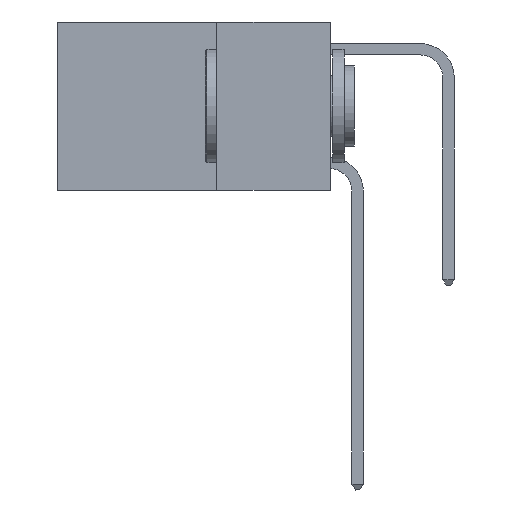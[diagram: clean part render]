
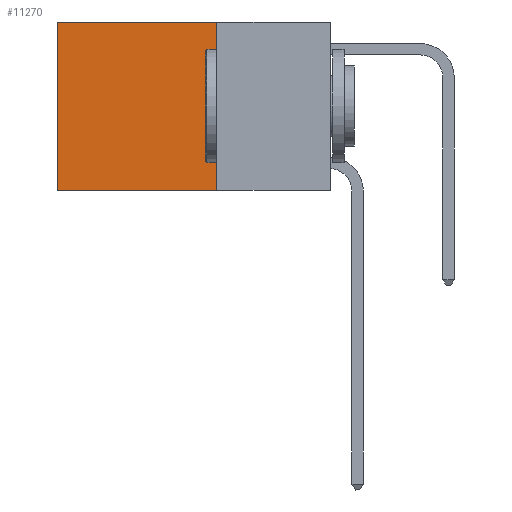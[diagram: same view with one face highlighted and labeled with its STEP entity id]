
A CAD part, left-side view. The second image highlights one B-rep face of the part: STEP entity #11270.
In plain terms, the highlighted planar face has unit normal (-1, 0, 0).
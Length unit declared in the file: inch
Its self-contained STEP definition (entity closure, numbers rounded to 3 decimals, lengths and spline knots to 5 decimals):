
#878 = DIRECTION ( 'NONE',  ( 1., 0., 0. ) ) ;
#1355 = ORIENTED_EDGE ( 'NONE', *, *, #2748, .T. ) ;
#2748 = EDGE_CURVE ( 'NONE', #13776, #4436, #9092, .T. ) ;
#3524 = EDGE_CURVE ( 'NONE', #13776, #14113, #11293, .T. ) ;
#4199 = CARTESIAN_POINT ( 'NONE',  ( 0.2625, 0.25, 0. ) ) ;
#4202 = DIRECTION ( 'NONE',  ( 0., 0., -1. ) ) ;
#4373 = VECTOR ( 'NONE', #18353, 39.37008 ) ;
#4436 = VERTEX_POINT ( 'NONE', #5403 ) ;
#4702 = CARTESIAN_POINT ( 'NONE',  ( 0.2625, 0.6, -0.37 ) ) ;
#5315 = VECTOR ( 'NONE', #4202, 39.37008 ) ;
#5403 = CARTESIAN_POINT ( 'NONE',  ( 0.2625, 0.6, 0. ) ) ;
#5965 = ORIENTED_EDGE ( 'NONE', *, *, #11442, .F. ) ;
#6932 = DIRECTION ( 'NONE',  ( 0., 0., -1. ) ) ;
#7676 = DIRECTION ( 'NONE',  ( 0., 0., -1. ) ) ;
#7707 = ORIENTED_EDGE ( 'NONE', *, *, #3524, .F. ) ;
#8050 = VECTOR ( 'NONE', #8995, 39.37008 ) ;
#8188 = CARTESIAN_POINT ( 'NONE',  ( 0.2625, 0.6, 0. ) ) ;
#8995 = DIRECTION ( 'NONE',  ( 0., 1., 0. ) ) ;
#9092 = LINE ( 'NONE', #9286, #8050 ) ;
#9260 = PLANE ( 'NONE',  #15032 ) ;
#9286 = CARTESIAN_POINT ( 'NONE',  ( 0.2625, 0.25, 0. ) ) ;
#9537 = LINE ( 'NONE', #11020, #4373 ) ;
#10552 = CARTESIAN_POINT ( 'NONE',  ( 0.2625, 0.25, 0. ) ) ;
#11020 = CARTESIAN_POINT ( 'NONE',  ( 0.2625, 0.25, -0.37 ) ) ;
#11270 = ADVANCED_FACE ( 'NONE', ( #17699 ), #9260, .F. ) ;
#11293 = LINE ( 'NONE', #14150, #18311 ) ;
#11442 = EDGE_CURVE ( 'NONE', #14113, #13022, #9537, .T. ) ;
#13022 = VERTEX_POINT ( 'NONE', #4702 ) ;
#13741 = LINE ( 'NONE', #8188, #5315 ) ;
#13776 = VERTEX_POINT ( 'NONE', #4199 ) ;
#14113 = VERTEX_POINT ( 'NONE', #16410 ) ;
#14150 = CARTESIAN_POINT ( 'NONE',  ( 0.2625, 0.25, 0. ) ) ;
#15028 = EDGE_CURVE ( 'NONE', #4436, #13022, #13741, .T. ) ;
#15032 = AXIS2_PLACEMENT_3D ( 'NONE', #10552, #878, #7676 ) ;
#16055 = ORIENTED_EDGE ( 'NONE', *, *, #15028, .T. ) ;
#16410 = CARTESIAN_POINT ( 'NONE',  ( 0.2625, 0.25, -0.37 ) ) ;
#17312 = EDGE_LOOP ( 'NONE', ( #16055, #5965, #7707, #1355 ) ) ;
#17699 = FACE_OUTER_BOUND ( 'NONE', #17312, .T. ) ;
#18311 = VECTOR ( 'NONE', #6932, 39.37008 ) ;
#18353 = DIRECTION ( 'NONE',  ( 0., 1., 0. ) ) ;
